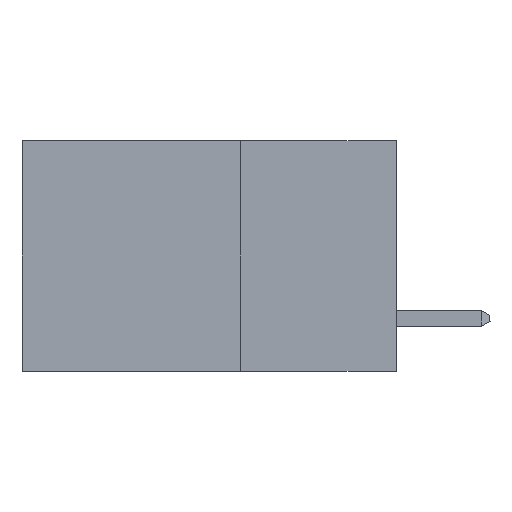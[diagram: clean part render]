
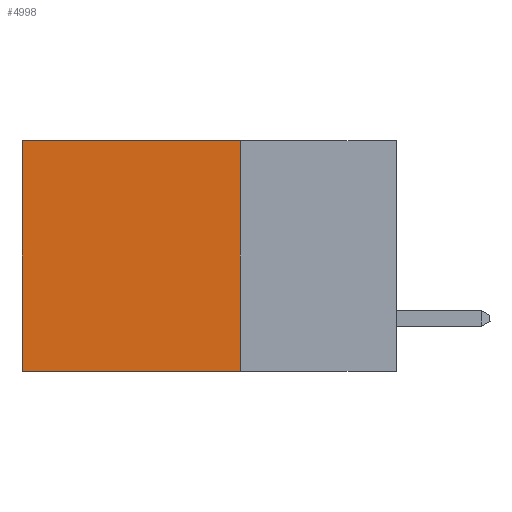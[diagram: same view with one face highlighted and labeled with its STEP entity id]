
A CAD part, left-side view. The second image highlights one B-rep face of the part: STEP entity #4998.
In plain terms, the highlighted planar face has unit normal (-1, 0, 0).
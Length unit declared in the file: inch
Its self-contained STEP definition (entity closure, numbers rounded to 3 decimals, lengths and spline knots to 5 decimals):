
#312 = VECTOR ( 'NONE', #2499, 39.37008 ) ;
#762 = EDGE_CURVE ( 'NONE', #4298, #6193, #973, .T. ) ;
#805 = DIRECTION ( 'NONE',  ( 0., 0., -1. ) ) ;
#973 = LINE ( 'NONE', #7403, #312 ) ;
#1192 = ORIENTED_EDGE ( 'NONE', *, *, #5530, .F. ) ;
#1484 = FACE_OUTER_BOUND ( 'NONE', #4862, .T. ) ;
#1912 = CARTESIAN_POINT ( 'NONE',  ( 0.298, 0.25, 0. ) ) ;
#2097 = DIRECTION ( 'NONE',  ( 0., 0., -1. ) ) ;
#2379 = VECTOR ( 'NONE', #2097, 39.37008 ) ;
#2494 = EDGE_CURVE ( 'NONE', #2887, #6193, #13007, .T. ) ;
#2499 = DIRECTION ( 'NONE',  ( 0., 1., 0. ) ) ;
#2678 = DIRECTION ( 'NONE',  ( 0., 0., -1. ) ) ;
#2887 = VERTEX_POINT ( 'NONE', #8958 ) ;
#4298 = VERTEX_POINT ( 'NONE', #7076 ) ;
#4862 = EDGE_LOOP ( 'NONE', ( #11705, #8867, #1192, #12806 ) ) ;
#4998 = ADVANCED_FACE ( 'NONE', ( #1484 ), #10154, .F. ) ;
#5266 = CARTESIAN_POINT ( 'NONE',  ( 0.298, 0.6, 0. ) ) ;
#5530 = EDGE_CURVE ( 'NONE', #9179, #4298, #11489, .T. ) ;
#5628 = CARTESIAN_POINT ( 'NONE',  ( 0.298, 0.25, 0. ) ) ;
#6193 = VERTEX_POINT ( 'NONE', #8933 ) ;
#6696 = DIRECTION ( 'NONE',  ( 0., 1., 0. ) ) ;
#7076 = CARTESIAN_POINT ( 'NONE',  ( 0.298, 0.25, -0.37 ) ) ;
#7149 = DIRECTION ( 'NONE',  ( 1., 0., 0. ) ) ;
#7403 = CARTESIAN_POINT ( 'NONE',  ( 0.298, 0.25, -0.37 ) ) ;
#8485 = VECTOR ( 'NONE', #2678, 39.37008 ) ;
#8867 = ORIENTED_EDGE ( 'NONE', *, *, #762, .F. ) ;
#8933 = CARTESIAN_POINT ( 'NONE',  ( 0.298, 0.6, -0.37 ) ) ;
#8958 = CARTESIAN_POINT ( 'NONE',  ( 0.298, 0.6, 0. ) ) ;
#9179 = VERTEX_POINT ( 'NONE', #1912 ) ;
#9912 = CARTESIAN_POINT ( 'NONE',  ( 0.298, 0.25, 0. ) ) ;
#10154 = PLANE ( 'NONE',  #11409 ) ;
#10529 = LINE ( 'NONE', #5628, #12912 ) ;
#10979 = EDGE_CURVE ( 'NONE', #9179, #2887, #10529, .T. ) ;
#11409 = AXIS2_PLACEMENT_3D ( 'NONE', #13197, #7149, #805 ) ;
#11489 = LINE ( 'NONE', #9912, #8485 ) ;
#11705 = ORIENTED_EDGE ( 'NONE', *, *, #2494, .T. ) ;
#12806 = ORIENTED_EDGE ( 'NONE', *, *, #10979, .T. ) ;
#12912 = VECTOR ( 'NONE', #6696, 39.37008 ) ;
#13007 = LINE ( 'NONE', #5266, #2379 ) ;
#13197 = CARTESIAN_POINT ( 'NONE',  ( 0.298, 0.25, 0. ) ) ;
